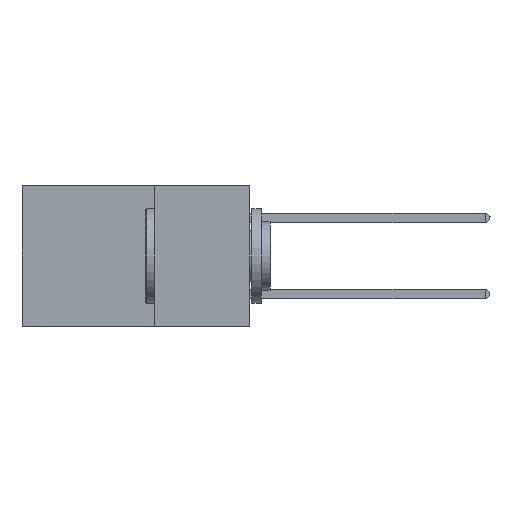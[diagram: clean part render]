
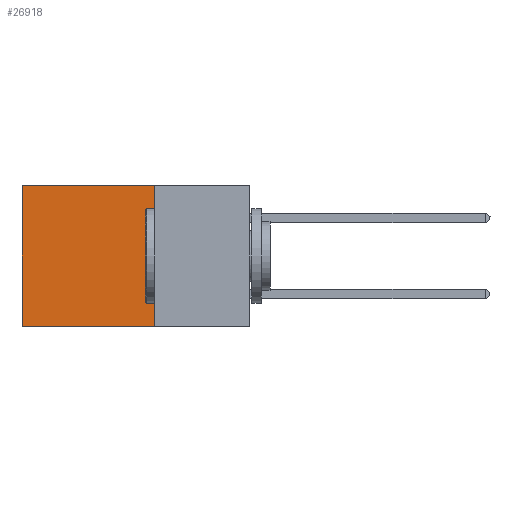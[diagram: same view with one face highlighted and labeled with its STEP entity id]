
A CAD part, left-side view. The second image highlights one B-rep face of the part: STEP entity #26918.
In plain terms, the highlighted planar face has unit normal (-1, 0, 0).
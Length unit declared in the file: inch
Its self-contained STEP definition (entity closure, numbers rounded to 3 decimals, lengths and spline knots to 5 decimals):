
#488 = VERTEX_POINT ( 'NONE', #8237 ) ;
#2082 = CARTESIAN_POINT ( 'NONE',  ( 0.2875, 0.25, 0. ) ) ;
#2660 = VECTOR ( 'NONE', #24272, 39.37008 ) ;
#2834 = EDGE_LOOP ( 'NONE', ( #13949, #27711, #9551, #30086 ) ) ;
#2837 = CARTESIAN_POINT ( 'NONE',  ( 0.2875, 0.25, 0. ) ) ;
#3168 = FACE_OUTER_BOUND ( 'NONE', #2834, .T. ) ;
#3714 = LINE ( 'NONE', #4693, #19608 ) ;
#4693 = CARTESIAN_POINT ( 'NONE',  ( 0.2875, 0.25, -0.37 ) ) ;
#6020 = DIRECTION ( 'NONE',  ( 1., 0., 0. ) ) ;
#7858 = DIRECTION ( 'NONE',  ( 0., 1., 0. ) ) ;
#8237 = CARTESIAN_POINT ( 'NONE',  ( 0.2875, 0.6, 0. ) ) ;
#8327 = CARTESIAN_POINT ( 'NONE',  ( 0.2875, 0.6, 0. ) ) ;
#8561 = EDGE_CURVE ( 'NONE', #35150, #488, #21596, .T. ) ;
#8595 = DIRECTION ( 'NONE',  ( 0., 1., 0. ) ) ;
#9551 = ORIENTED_EDGE ( 'NONE', *, *, #21488, .F. ) ;
#10658 = CARTESIAN_POINT ( 'NONE',  ( 0.2875, 0.6, -0.37 ) ) ;
#12095 = CARTESIAN_POINT ( 'NONE',  ( 0.2875, 0.25, 0. ) ) ;
#12104 = EDGE_CURVE ( 'NONE', #28515, #30611, #3714, .T. ) ;
#13949 = ORIENTED_EDGE ( 'NONE', *, *, #35137, .T. ) ;
#18694 = PLANE ( 'NONE',  #38603 ) ;
#18965 = LINE ( 'NONE', #12095, #33722 ) ;
#19608 = VECTOR ( 'NONE', #7858, 39.37008 ) ;
#21488 = EDGE_CURVE ( 'NONE', #35150, #28515, #18965, .T. ) ;
#21596 = LINE ( 'NONE', #33858, #37222 ) ;
#24272 = DIRECTION ( 'NONE',  ( 0., 0., -1. ) ) ;
#24818 = DIRECTION ( 'NONE',  ( 0., 0., -1. ) ) ;
#26918 = ADVANCED_FACE ( 'NONE', ( #3168 ), #18694, .F. ) ;
#27711 = ORIENTED_EDGE ( 'NONE', *, *, #12104, .F. ) ;
#27920 = LINE ( 'NONE', #8327, #2660 ) ;
#28175 = DIRECTION ( 'NONE',  ( 0., 0., -1. ) ) ;
#28515 = VERTEX_POINT ( 'NONE', #35564 ) ;
#30086 = ORIENTED_EDGE ( 'NONE', *, *, #8561, .T. ) ;
#30611 = VERTEX_POINT ( 'NONE', #10658 ) ;
#33722 = VECTOR ( 'NONE', #24818, 39.37008 ) ;
#33858 = CARTESIAN_POINT ( 'NONE',  ( 0.2875, 0.25, 0. ) ) ;
#35137 = EDGE_CURVE ( 'NONE', #488, #30611, #27920, .T. ) ;
#35150 = VERTEX_POINT ( 'NONE', #2082 ) ;
#35564 = CARTESIAN_POINT ( 'NONE',  ( 0.2875, 0.25, -0.37 ) ) ;
#37222 = VECTOR ( 'NONE', #8595, 39.37008 ) ;
#38603 = AXIS2_PLACEMENT_3D ( 'NONE', #2837, #6020, #28175 ) ;
